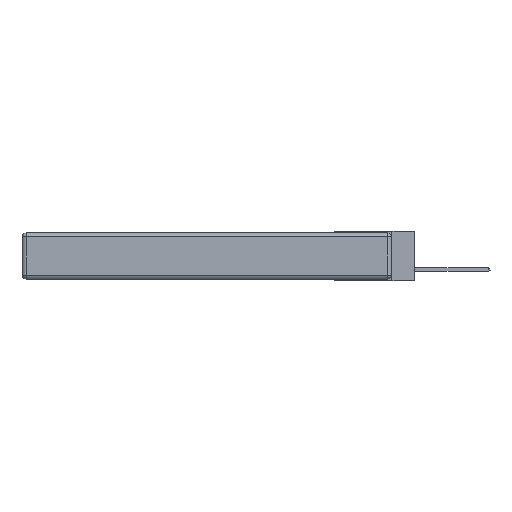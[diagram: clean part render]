
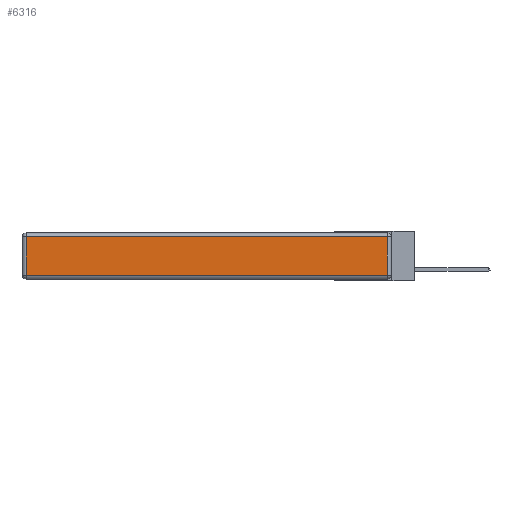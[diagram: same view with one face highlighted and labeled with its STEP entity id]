
A CAD part, left-side view. The second image highlights one B-rep face of the part: STEP entity #6316.
In plain terms, the highlighted planar face has unit normal (-1, 0, 0).
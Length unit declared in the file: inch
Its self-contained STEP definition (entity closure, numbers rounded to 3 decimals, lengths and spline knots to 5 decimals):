
#835 = LINE ( 'NONE', #6170, #5622 ) ;
#1397 = DIRECTION ( 'NONE',  ( 0., 0., 1. ) ) ;
#2007 = PLANE ( 'NONE',  #5576 ) ;
#2860 = DIRECTION ( 'NONE',  ( 0., 0., 1. ) ) ;
#2956 = EDGE_CURVE ( 'NONE', #10442, #7579, #5499, .T. ) ;
#3024 = CARTESIAN_POINT ( 'NONE',  ( 0., 0.03, -0.313 ) ) ;
#3841 = VERTEX_POINT ( 'NONE', #7841 ) ;
#3851 = DIRECTION ( 'NONE',  ( 0., 1., 0. ) ) ;
#3884 = EDGE_CURVE ( 'NONE', #3841, #8362, #7391, .T. ) ;
#4032 = ORIENTED_EDGE ( 'NONE', *, *, #3884, .T. ) ;
#4497 = VECTOR ( 'NONE', #1397, 39.37008 ) ;
#5499 = LINE ( 'NONE', #6970, #4497 ) ;
#5557 = DIRECTION ( 'NONE',  ( -1., 0., 0. ) ) ;
#5576 = AXIS2_PLACEMENT_3D ( 'NONE', #8372, #5557, #2860 ) ;
#5622 = VECTOR ( 'NONE', #9920, 39.37008 ) ;
#6170 = CARTESIAN_POINT ( 'NONE',  ( 0., 0., -0.313 ) ) ;
#6177 = FACE_OUTER_BOUND ( 'NONE', #6586, .T. ) ;
#6296 = EDGE_CURVE ( 'NONE', #7579, #3841, #6908, .T. ) ;
#6316 = ADVANCED_FACE ( 'NONE', ( #6177 ), #2007, .T. ) ;
#6365 = VECTOR ( 'NONE', #10279, 39.37008 ) ;
#6586 = EDGE_LOOP ( 'NONE', ( #8855, #8962, #9532, #4032 ) ) ;
#6629 = CARTESIAN_POINT ( 'NONE',  ( 0., 2.75, -0.03 ) ) ;
#6908 = LINE ( 'NONE', #6629, #7943 ) ;
#6970 = CARTESIAN_POINT ( 'NONE',  ( 0., 0.03, -0.343 ) ) ;
#7391 = LINE ( 'NONE', #10615, #6365 ) ;
#7577 = EDGE_CURVE ( 'NONE', #8362, #10442, #835, .T. ) ;
#7579 = VERTEX_POINT ( 'NONE', #8062 ) ;
#7841 = CARTESIAN_POINT ( 'NONE',  ( 0., 2.72, -0.03 ) ) ;
#7943 = VECTOR ( 'NONE', #3851, 39.37008 ) ;
#8062 = CARTESIAN_POINT ( 'NONE',  ( 0., 0.03, -0.03 ) ) ;
#8362 = VERTEX_POINT ( 'NONE', #9025 ) ;
#8372 = CARTESIAN_POINT ( 'NONE',  ( 0., 0., -0.343 ) ) ;
#8855 = ORIENTED_EDGE ( 'NONE', *, *, #7577, .T. ) ;
#8962 = ORIENTED_EDGE ( 'NONE', *, *, #2956, .T. ) ;
#9025 = CARTESIAN_POINT ( 'NONE',  ( 0., 2.72, -0.313 ) ) ;
#9532 = ORIENTED_EDGE ( 'NONE', *, *, #6296, .T. ) ;
#9920 = DIRECTION ( 'NONE',  ( 0., -1., 0. ) ) ;
#10279 = DIRECTION ( 'NONE',  ( 0., 0., -1. ) ) ;
#10442 = VERTEX_POINT ( 'NONE', #3024 ) ;
#10615 = CARTESIAN_POINT ( 'NONE',  ( 0., 2.72, -0.343 ) ) ;
